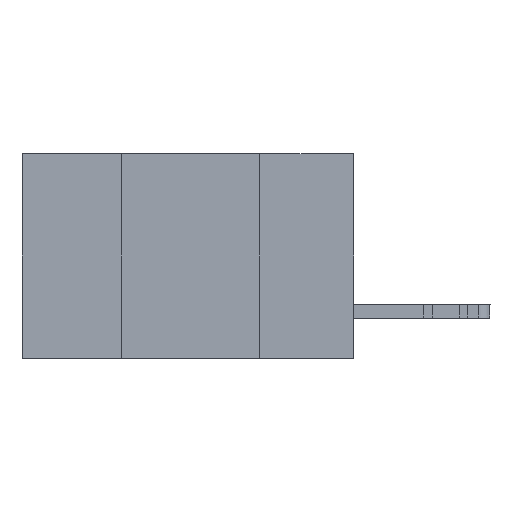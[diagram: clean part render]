
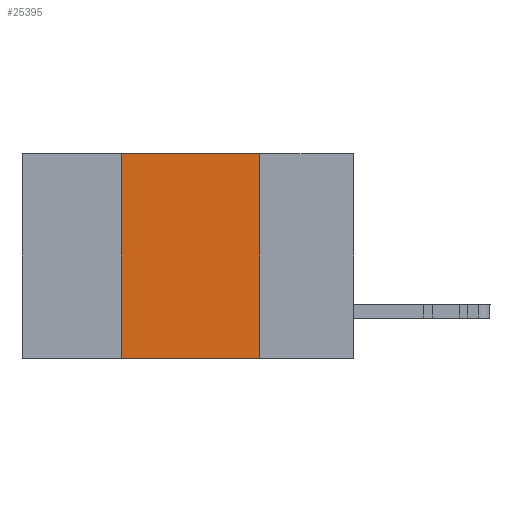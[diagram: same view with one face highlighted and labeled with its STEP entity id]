
A CAD part, left-side view. The second image highlights one B-rep face of the part: STEP entity #25395.
In plain terms, the highlighted planar face has unit normal (-1, 0, 0).
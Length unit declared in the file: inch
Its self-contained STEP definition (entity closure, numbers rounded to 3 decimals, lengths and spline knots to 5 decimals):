
#332 = CARTESIAN_POINT ( 'NONE',  ( 0., 0.17, 0. ) ) ;
#338 = VECTOR ( 'NONE', #37119, 39.37008 ) ;
#1376 = EDGE_CURVE ( 'NONE', #13204, #41486, #28211, .T. ) ;
#1453 = ORIENTED_EDGE ( 'NONE', *, *, #9108, .F. ) ;
#1470 = EDGE_CURVE ( 'NONE', #14361, #41486, #11443, .T. ) ;
#3855 = PLANE ( 'NONE',  #22279 ) ;
#3924 = LINE ( 'NONE', #21986, #25564 ) ;
#7082 = ORIENTED_EDGE ( 'NONE', *, *, #1376, .T. ) ;
#8175 = CARTESIAN_POINT ( 'NONE',  ( 0., 0.42, -0.37 ) ) ;
#8808 = CARTESIAN_POINT ( 'NONE',  ( 0., 0.6, 0. ) ) ;
#9108 = EDGE_CURVE ( 'NONE', #45798, #14361, #36668, .T. ) ;
#9316 = EDGE_CURVE ( 'NONE', #13204, #45798, #3924, .T. ) ;
#10877 = DIRECTION ( 'NONE',  ( 0., 0., 1. ) ) ;
#11252 = DIRECTION ( 'NONE',  ( 0., 0., -1. ) ) ;
#11443 = LINE ( 'NONE', #332, #23553 ) ;
#13204 = VERTEX_POINT ( 'NONE', #8175 ) ;
#14067 = FACE_OUTER_BOUND ( 'NONE', #28322, .T. ) ;
#14361 = VERTEX_POINT ( 'NONE', #40820 ) ;
#17062 = DIRECTION ( 'NONE',  ( 0., -1., 0. ) ) ;
#21986 = CARTESIAN_POINT ( 'NONE',  ( 0., 0.42, 0. ) ) ;
#22279 = AXIS2_PLACEMENT_3D ( 'NONE', #42436, #39154, #11252 ) ;
#23553 = VECTOR ( 'NONE', #42620, 39.37008 ) ;
#25395 = ADVANCED_FACE ( 'NONE', ( #14067 ), #3855, .F. ) ;
#25398 = CARTESIAN_POINT ( 'NONE',  ( 0., 0.17, -0.37 ) ) ;
#25564 = VECTOR ( 'NONE', #10877, 39.37008 ) ;
#26770 = ORIENTED_EDGE ( 'NONE', *, *, #9316, .F. ) ;
#27517 = CARTESIAN_POINT ( 'NONE',  ( 0., 0.6, -0.37 ) ) ;
#28043 = VECTOR ( 'NONE', #17062, 39.37008 ) ;
#28211 = LINE ( 'NONE', #27517, #28043 ) ;
#28322 = EDGE_LOOP ( 'NONE', ( #34567, #1453, #26770, #7082 ) ) ;
#28634 = CARTESIAN_POINT ( 'NONE',  ( 0., 0.42, 0. ) ) ;
#34567 = ORIENTED_EDGE ( 'NONE', *, *, #1470, .F. ) ;
#36668 = LINE ( 'NONE', #8808, #338 ) ;
#37119 = DIRECTION ( 'NONE',  ( 0., -1., 0. ) ) ;
#39154 = DIRECTION ( 'NONE',  ( 1., 0., 0. ) ) ;
#40820 = CARTESIAN_POINT ( 'NONE',  ( 0., 0.17, 0. ) ) ;
#41486 = VERTEX_POINT ( 'NONE', #25398 ) ;
#42436 = CARTESIAN_POINT ( 'NONE',  ( 0., 0.6, 0. ) ) ;
#42620 = DIRECTION ( 'NONE',  ( 0., 0., -1. ) ) ;
#45798 = VERTEX_POINT ( 'NONE', #28634 ) ;
